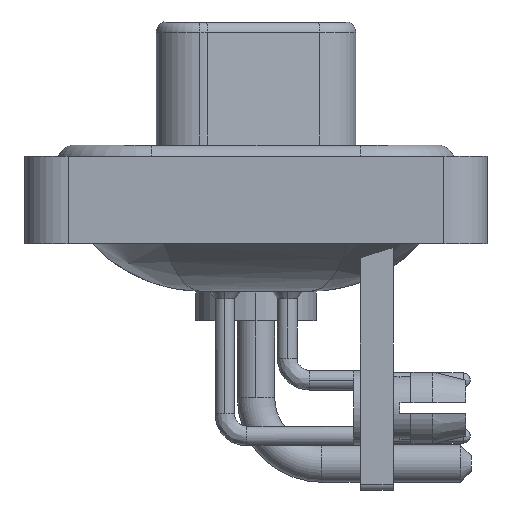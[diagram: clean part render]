
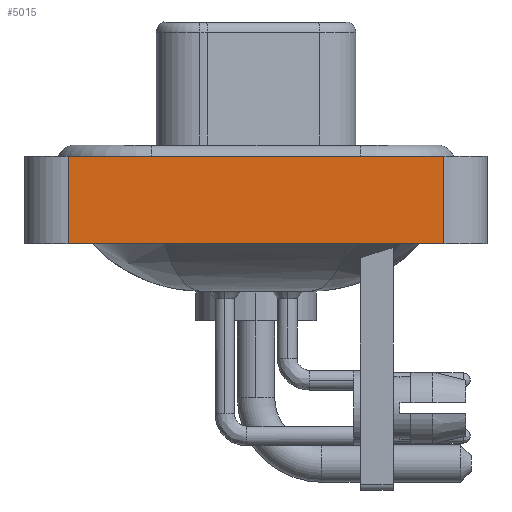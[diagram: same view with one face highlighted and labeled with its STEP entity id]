
A CAD part, left-side view. The second image highlights one B-rep face of the part: STEP entity #5015.
In plain terms, the highlighted planar face has unit normal (-1, 0, 0).
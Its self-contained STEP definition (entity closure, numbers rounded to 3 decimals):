
#23 = VECTOR ( 'NONE', #23291, 1000. ) ;
#51 = AXIS2_PLACEMENT_3D ( 'NONE', #10963, #26600, #11371 ) ;
#317 = DIRECTION ( 'NONE',  ( 0., 0., 1. ) ) ;
#401 = EDGE_CURVE ( 'NONE', #5025, #21223, #11175, .T. ) ;
#1726 = EDGE_CURVE ( 'NONE', #27084, #26238, #23988, .T. ) ;
#2269 = PLANE ( 'NONE',  #51 ) ;
#2530 = CARTESIAN_POINT ( 'NONE',  ( -7.3, -8.55, -3.6 ) ) ;
#2672 = VECTOR ( 'NONE', #10933, 1000. ) ;
#3872 = EDGE_LOOP ( 'NONE', ( #15787, #19002, #7984, #7830 ) ) ;
#4613 = CARTESIAN_POINT ( 'NONE',  ( -7.3, 8.55, 0.4 ) ) ;
#5015 = ADVANCED_FACE ( 'NONE', ( #20235 ), #2269, .T. ) ;
#5019 = CARTESIAN_POINT ( 'NONE',  ( -7.3, -8.55, -3.6 ) ) ;
#5025 = VERTEX_POINT ( 'NONE', #2530 ) ;
#5213 = CARTESIAN_POINT ( 'NONE',  ( -7.3, -8.55, -3.6 ) ) ;
#7830 = ORIENTED_EDGE ( 'NONE', *, *, #17867, .T. ) ;
#7984 = ORIENTED_EDGE ( 'NONE', *, *, #1726, .F. ) ;
#8538 = CARTESIAN_POINT ( 'NONE',  ( -7.3, -8.55, 0.4 ) ) ;
#9779 = CARTESIAN_POINT ( 'NONE',  ( -7.3, 8.55, -3.6 ) ) ;
#10933 = DIRECTION ( 'NONE',  ( 0., 0., 1. ) ) ;
#10963 = CARTESIAN_POINT ( 'NONE',  ( -7.3, -8.55, -3.6 ) ) ;
#11175 = LINE ( 'NONE', #5019, #25916 ) ;
#11371 = DIRECTION ( 'NONE',  ( 0., 0., 1. ) ) ;
#13481 = VECTOR ( 'NONE', #23120, 1000. ) ;
#14506 = LINE ( 'NONE', #8538, #23 ) ;
#15787 = ORIENTED_EDGE ( 'NONE', *, *, #401, .T. ) ;
#17867 = EDGE_CURVE ( 'NONE', #27084, #5025, #18672, .T. ) ;
#18672 = LINE ( 'NONE', #5213, #13481 ) ;
#19002 = ORIENTED_EDGE ( 'NONE', *, *, #19869, .F. ) ;
#19869 = EDGE_CURVE ( 'NONE', #26238, #21223, #14506, .T. ) ;
#20235 = FACE_OUTER_BOUND ( 'NONE', #3872, .T. ) ;
#21223 = VERTEX_POINT ( 'NONE', #27548 ) ;
#21841 = CARTESIAN_POINT ( 'NONE',  ( -7.3, 8.55, -3.6 ) ) ;
#23120 = DIRECTION ( 'NONE',  ( 0., -1., 0. ) ) ;
#23291 = DIRECTION ( 'NONE',  ( 0., -1., 0. ) ) ;
#23988 = LINE ( 'NONE', #21841, #2672 ) ;
#25916 = VECTOR ( 'NONE', #317, 1000. ) ;
#26238 = VERTEX_POINT ( 'NONE', #4613 ) ;
#26600 = DIRECTION ( 'NONE',  ( -1., 0., 0. ) ) ;
#27084 = VERTEX_POINT ( 'NONE', #9779 ) ;
#27548 = CARTESIAN_POINT ( 'NONE',  ( -7.3, -8.55, 0.4 ) ) ;
